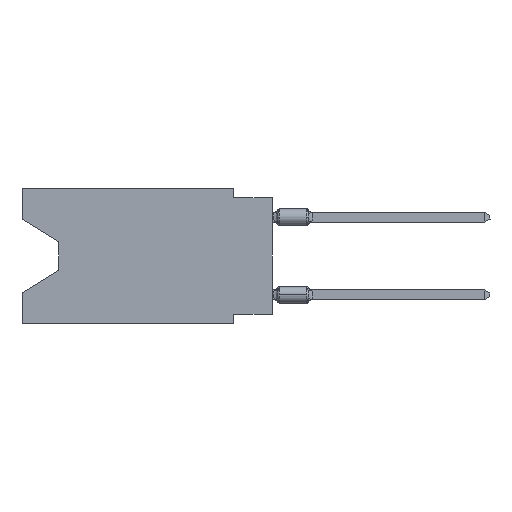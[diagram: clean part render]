
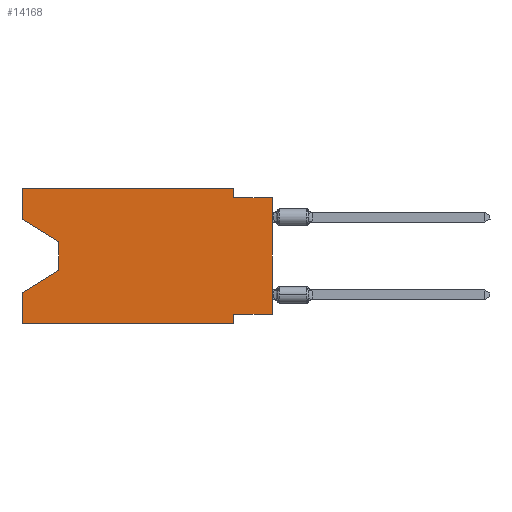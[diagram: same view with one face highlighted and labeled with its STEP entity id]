
A CAD part, left-side view. The second image highlights one B-rep face of the part: STEP entity #14168.
In plain terms, the highlighted planar face has unit normal (-1, 0, 0).
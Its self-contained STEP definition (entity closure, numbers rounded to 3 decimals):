
#26 = EDGE_LOOP ( 'NONE', ( #27374, #1119, #39697, #10090, #6748, #26730, #29073, #36904, #13540, #6164, #19304, #14386 ) ) ;
#200 = CARTESIAN_POINT ( 'NONE',  ( 0., 16.383, -2.038 ) ) ;
#209 = VERTEX_POINT ( 'NONE', #12753 ) ;
#277 = LINE ( 'NONE', #10170, #41410 ) ;
#304 = LINE ( 'NONE', #14024, #17945 ) ;
#446 = VECTOR ( 'NONE', #33908, 1000. ) ;
#1119 = ORIENTED_EDGE ( 'NONE', *, *, #39092, .T. ) ;
#1246 = LINE ( 'NONE', #14971, #34265 ) ;
#2215 = VECTOR ( 'NONE', #5449, 1000. ) ;
#3433 = DIRECTION ( 'NONE',  ( 0., 0., 1. ) ) ;
#3566 = CARTESIAN_POINT ( 'NONE',  ( 0., 0., -8.255 ) ) ;
#4145 = VERTEX_POINT ( 'NONE', #36787 ) ;
#4270 = EDGE_CURVE ( 'NONE', #4145, #23411, #304, .T. ) ;
#4663 = VECTOR ( 'NONE', #28732, 1000. ) ;
#5213 = DIRECTION ( 'NONE',  ( 0., 0., 1. ) ) ;
#5449 = DIRECTION ( 'NONE',  ( 0., 0.855, -0.519 ) ) ;
#6012 = LINE ( 'NONE', #43325, #7481 ) ;
#6039 = EDGE_CURVE ( 'NONE', #40380, #26671, #25061, .T. ) ;
#6164 = ORIENTED_EDGE ( 'NONE', *, *, #17022, .F. ) ;
#6748 = ORIENTED_EDGE ( 'NONE', *, *, #38345, .T. ) ;
#7481 = VECTOR ( 'NONE', #22437, 1000. ) ;
#7534 = CARTESIAN_POINT ( 'NONE',  ( 0., 2.54, 0. ) ) ;
#8490 = LINE ( 'NONE', #35897, #4663 ) ;
#8535 = VECTOR ( 'NONE', #5213, 1000. ) ;
#8581 = CARTESIAN_POINT ( 'NONE',  ( 0., 16.383, 0. ) ) ;
#10090 = ORIENTED_EDGE ( 'NONE', *, *, #27157, .F. ) ;
#10170 = CARTESIAN_POINT ( 'NONE',  ( 0., 16.383, 0. ) ) ;
#11013 = EDGE_CURVE ( 'NONE', #17610, #11102, #15337, .T. ) ;
#11102 = VERTEX_POINT ( 'NONE', #22520 ) ;
#11578 = VERTEX_POINT ( 'NONE', #19095 ) ;
#12753 = CARTESIAN_POINT ( 'NONE',  ( 0., 13.97, -5.385 ) ) ;
#13540 = ORIENTED_EDGE ( 'NONE', *, *, #4270, .F. ) ;
#13950 = CARTESIAN_POINT ( 'NONE',  ( 0., 2.54, -8.89 ) ) ;
#14024 = CARTESIAN_POINT ( 'NONE',  ( 0., 0., -0.635 ) ) ;
#14168 = ADVANCED_FACE ( 'NONE', ( #41319 ), #37489, .F. ) ;
#14386 = ORIENTED_EDGE ( 'NONE', *, *, #11013, .F. ) ;
#14971 = CARTESIAN_POINT ( 'NONE',  ( 0., 13.97, -3.505 ) ) ;
#15337 = LINE ( 'NONE', #8581, #8535 ) ;
#15795 = CARTESIAN_POINT ( 'NONE',  ( 0., 13.97, -5.385 ) ) ;
#16251 = VERTEX_POINT ( 'NONE', #40218 ) ;
#16668 = EDGE_CURVE ( 'NONE', #17610, #16251, #6012, .T. ) ;
#16800 = CARTESIAN_POINT ( 'NONE',  ( 0., 2.54, -8.255 ) ) ;
#16839 = DIRECTION ( 'NONE',  ( 0., 0., -1. ) ) ;
#17022 = EDGE_CURVE ( 'NONE', #26779, #4145, #30617, .T. ) ;
#17610 = VERTEX_POINT ( 'NONE', #200 ) ;
#17945 = VECTOR ( 'NONE', #38518, 1000. ) ;
#18302 = VECTOR ( 'NONE', #33971, 1000. ) ;
#19095 = CARTESIAN_POINT ( 'NONE',  ( 0., 2.54, -8.89 ) ) ;
#19304 = ORIENTED_EDGE ( 'NONE', *, *, #30758, .F. ) ;
#19488 = VECTOR ( 'NONE', #35016, 1000. ) ;
#20061 = CARTESIAN_POINT ( 'NONE',  ( 0., 2.54, 0. ) ) ;
#21896 = CARTESIAN_POINT ( 'NONE',  ( 0., 0., -0.635 ) ) ;
#22437 = DIRECTION ( 'NONE',  ( 0., -0.855, -0.519 ) ) ;
#22520 = CARTESIAN_POINT ( 'NONE',  ( 0., 16.383, 0. ) ) ;
#23411 = VERTEX_POINT ( 'NONE', #21896 ) ;
#24246 = CARTESIAN_POINT ( 'NONE',  ( 0., 16.383, 0. ) ) ;
#24599 = CARTESIAN_POINT ( 'NONE',  ( 0., 0., -8.255 ) ) ;
#25061 = LINE ( 'NONE', #24599, #25985 ) ;
#25985 = VECTOR ( 'NONE', #28424, 1000. ) ;
#26671 = VERTEX_POINT ( 'NONE', #16800 ) ;
#26730 = ORIENTED_EDGE ( 'NONE', *, *, #35583, .F. ) ;
#26779 = VERTEX_POINT ( 'NONE', #7534 ) ;
#27157 = EDGE_CURVE ( 'NONE', #41635, #43069, #277, .T. ) ;
#27374 = ORIENTED_EDGE ( 'NONE', *, *, #16668, .T. ) ;
#28079 = CARTESIAN_POINT ( 'NONE',  ( 0., 16.383, -8.89 ) ) ;
#28318 = VECTOR ( 'NONE', #41137, 1000. ) ;
#28424 = DIRECTION ( 'NONE',  ( 0., 1., 0. ) ) ;
#28732 = DIRECTION ( 'NONE',  ( 0., 0., 1. ) ) ;
#29073 = ORIENTED_EDGE ( 'NONE', *, *, #6039, .F. ) ;
#30119 = LINE ( 'NONE', #36842, #446 ) ;
#30259 = EDGE_CURVE ( 'NONE', #209, #43069, #38950, .T. ) ;
#30586 = LINE ( 'NONE', #13950, #28318 ) ;
#30617 = LINE ( 'NONE', #20061, #18302 ) ;
#30758 = EDGE_CURVE ( 'NONE', #11102, #26779, #31416, .T. ) ;
#31416 = LINE ( 'NONE', #24246, #19488 ) ;
#33217 = CARTESIAN_POINT ( 'NONE',  ( 0., 16.383, 0. ) ) ;
#33908 = DIRECTION ( 'NONE',  ( 0., -1., 0. ) ) ;
#33971 = DIRECTION ( 'NONE',  ( 0., 0., -1. ) ) ;
#34265 = VECTOR ( 'NONE', #37892, 1000. ) ;
#35016 = DIRECTION ( 'NONE',  ( 0., -1., 0. ) ) ;
#35583 = EDGE_CURVE ( 'NONE', #26671, #11578, #30586, .T. ) ;
#35897 = CARTESIAN_POINT ( 'NONE',  ( 0., 0., 0. ) ) ;
#36150 = EDGE_CURVE ( 'NONE', #40380, #23411, #8490, .T. ) ;
#36787 = CARTESIAN_POINT ( 'NONE',  ( 0., 2.54, -0.635 ) ) ;
#36842 = CARTESIAN_POINT ( 'NONE',  ( 0., 16.383, -8.89 ) ) ;
#36904 = ORIENTED_EDGE ( 'NONE', *, *, #36150, .T. ) ;
#37489 = PLANE ( 'NONE',  #44169 ) ;
#37892 = DIRECTION ( 'NONE',  ( 0., 0., -1. ) ) ;
#37943 = DIRECTION ( 'NONE',  ( 1., 0., 0. ) ) ;
#38345 = EDGE_CURVE ( 'NONE', #41635, #11578, #30119, .T. ) ;
#38518 = DIRECTION ( 'NONE',  ( 0., -1., 0. ) ) ;
#38950 = LINE ( 'NONE', #15795, #2215 ) ;
#39092 = EDGE_CURVE ( 'NONE', #16251, #209, #1246, .T. ) ;
#39697 = ORIENTED_EDGE ( 'NONE', *, *, #30259, .T. ) ;
#40218 = CARTESIAN_POINT ( 'NONE',  ( 0., 13.97, -3.505 ) ) ;
#40380 = VERTEX_POINT ( 'NONE', #3566 ) ;
#41137 = DIRECTION ( 'NONE',  ( 0., 0., -1. ) ) ;
#41319 = FACE_OUTER_BOUND ( 'NONE', #26, .T. ) ;
#41410 = VECTOR ( 'NONE', #3433, 1000. ) ;
#41635 = VERTEX_POINT ( 'NONE', #28079 ) ;
#43069 = VERTEX_POINT ( 'NONE', #44200 ) ;
#43325 = CARTESIAN_POINT ( 'NONE',  ( 0., 16.383, -2.038 ) ) ;
#44169 = AXIS2_PLACEMENT_3D ( 'NONE', #33217, #37943, #16839 ) ;
#44200 = CARTESIAN_POINT ( 'NONE',  ( 0., 16.383, -6.852 ) ) ;
